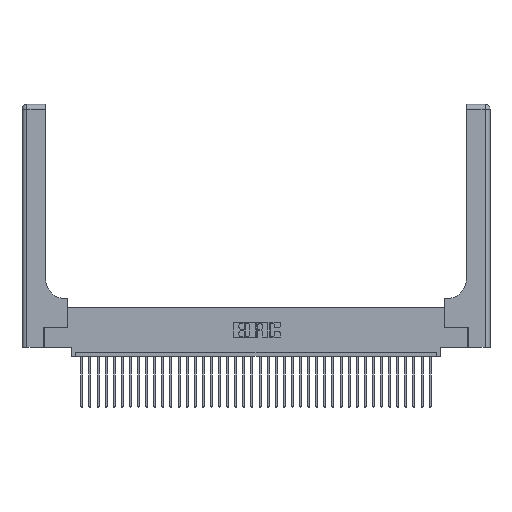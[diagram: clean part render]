
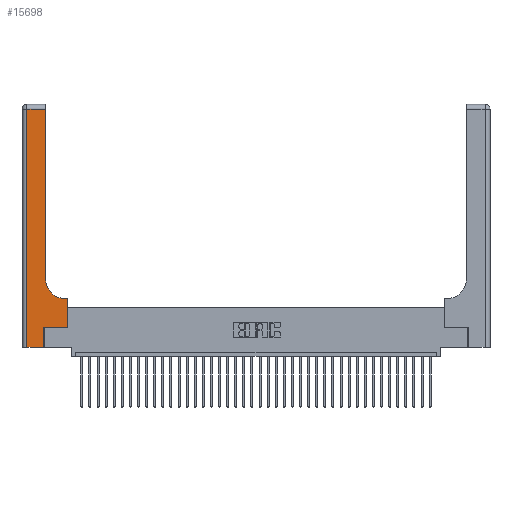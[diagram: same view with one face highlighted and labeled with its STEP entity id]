
A CAD part, top view. The second image highlights one B-rep face of the part: STEP entity #15698.
In plain terms, the highlighted planar face has unit normal (0, 0, 1).
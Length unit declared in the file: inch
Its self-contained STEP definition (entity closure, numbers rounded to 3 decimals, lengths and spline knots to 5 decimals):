
#1615 = ORIENTED_EDGE ( 'NONE', *, *, #35983, .T. ) ;
#2591 = VECTOR ( 'NONE', #10965, 39.37008 ) ;
#2613 = LINE ( 'NONE', #31323, #20630 ) ;
#2653 = CIRCLE ( 'NONE', #23347, 0.25 ) ;
#3253 = DIRECTION ( 'NONE',  ( 0., -1., 0. ) ) ;
#3875 = LINE ( 'NONE', #9169, #34372 ) ;
#4025 = CARTESIAN_POINT ( 'NONE',  ( 0.06, 2.94, 0.37 ) ) ;
#4198 = ORIENTED_EDGE ( 'NONE', *, *, #8417, .T. ) ;
#4744 = ORIENTED_EDGE ( 'NONE', *, *, #29244, .T. ) ;
#5102 = ORIENTED_EDGE ( 'NONE', *, *, #23853, .T. ) ;
#6579 = DIRECTION ( 'NONE',  ( 0., 1., 0. ) ) ;
#6632 = AXIS2_PLACEMENT_3D ( 'NONE', #10665, #25784, #16975 ) ;
#6956 = CARTESIAN_POINT ( 'NONE',  ( 0.2915, 2.94, 0.37 ) ) ;
#7447 = EDGE_CURVE ( 'NONE', #20373, #27268, #31253, .T. ) ;
#7867 = LINE ( 'NONE', #11156, #29525 ) ;
#7925 = DIRECTION ( 'NONE',  ( 0., 1., 0. ) ) ;
#7994 = CARTESIAN_POINT ( 'NONE',  ( 0., 0., 0.37 ) ) ;
#8121 = CARTESIAN_POINT ( 'NONE',  ( 0.5585, 0.25, 0.37 ) ) ;
#8356 = CARTESIAN_POINT ( 'NONE',  ( 0.269, 0.25, 0.37 ) ) ;
#8417 = EDGE_CURVE ( 'NONE', #19033, #24531, #37881, .T. ) ;
#9169 = CARTESIAN_POINT ( 'NONE',  ( 0.2915, 3., 0.37 ) ) ;
#9247 = VECTOR ( 'NONE', #31862, 39.37008 ) ;
#9699 = CARTESIAN_POINT ( 'NONE',  ( 0., 2.94, 0.37 ) ) ;
#10398 = VERTEX_POINT ( 'NONE', #6956 ) ;
#10665 = CARTESIAN_POINT ( 'NONE',  ( 0., 3., 0.37 ) ) ;
#10712 = EDGE_CURVE ( 'NONE', #16524, #20373, #2613, .T. ) ;
#10965 = DIRECTION ( 'NONE',  ( 1., 0., 0. ) ) ;
#11080 = EDGE_CURVE ( 'NONE', #20494, #18774, #17378, .T. ) ;
#11156 = CARTESIAN_POINT ( 'NONE',  ( 0.269, 0., 0.37 ) ) ;
#11181 = PLANE ( 'NONE',  #6632 ) ;
#12588 = EDGE_CURVE ( 'NONE', #24531, #20494, #32113, .T. ) ;
#12649 = DIRECTION ( 'NONE',  ( -1., 0., 0. ) ) ;
#12998 = CARTESIAN_POINT ( 'NONE',  ( 0.2915, 0.85, 0.37 ) ) ;
#14057 = VECTOR ( 'NONE', #34293, 39.37008 ) ;
#15144 = CARTESIAN_POINT ( 'NONE',  ( 0.5415, 0.6, 0.37 ) ) ;
#15698 = ADVANCED_FACE ( 'NONE', ( #36290 ), #11181, .F. ) ;
#16325 = DIRECTION ( 'NONE',  ( 0., 0., -1. ) ) ;
#16524 = VERTEX_POINT ( 'NONE', #4025 ) ;
#16700 = ORIENTED_EDGE ( 'NONE', *, *, #10712, .T. ) ;
#16975 = DIRECTION ( 'NONE',  ( -1., 0., 0. ) ) ;
#17378 = LINE ( 'NONE', #31148, #26608 ) ;
#17421 = ORIENTED_EDGE ( 'NONE', *, *, #30627, .T. ) ;
#17640 = CARTESIAN_POINT ( 'NONE',  ( 0.5585, 0.25, 0.37 ) ) ;
#18774 = VERTEX_POINT ( 'NONE', #15144 ) ;
#18900 = VERTEX_POINT ( 'NONE', #12998 ) ;
#19033 = VERTEX_POINT ( 'NONE', #27196 ) ;
#20373 = VERTEX_POINT ( 'NONE', #24460 ) ;
#20494 = VERTEX_POINT ( 'NONE', #28140 ) ;
#20630 = VECTOR ( 'NONE', #3253, 39.37008 ) ;
#22955 = LINE ( 'NONE', #9699, #30339 ) ;
#23347 = AXIS2_PLACEMENT_3D ( 'NONE', #31449, #16325, #34248 ) ;
#23853 = EDGE_CURVE ( 'NONE', #18900, #10398, #3875, .T. ) ;
#24460 = CARTESIAN_POINT ( 'NONE',  ( 0.06, 0., 0.37 ) ) ;
#24531 = VERTEX_POINT ( 'NONE', #17640 ) ;
#25506 = DIRECTION ( 'NONE',  ( -1., 0., 0. ) ) ;
#25784 = DIRECTION ( 'NONE',  ( 0., 0., -1. ) ) ;
#26002 = ORIENTED_EDGE ( 'NONE', *, *, #11080, .T. ) ;
#26049 = CARTESIAN_POINT ( 'NONE',  ( 0.269, 0., 0.37 ) ) ;
#26366 = EDGE_LOOP ( 'NONE', ( #5102, #1615, #16700, #33769, #4744, #4198, #27893, #26002, #17421 ) ) ;
#26608 = VECTOR ( 'NONE', #25506, 39.37008 ) ;
#27196 = CARTESIAN_POINT ( 'NONE',  ( 0.269, 0.25, 0.37 ) ) ;
#27268 = VERTEX_POINT ( 'NONE', #26049 ) ;
#27893 = ORIENTED_EDGE ( 'NONE', *, *, #12588, .T. ) ;
#28140 = CARTESIAN_POINT ( 'NONE',  ( 0.5585, 0.6, 0.37 ) ) ;
#29244 = EDGE_CURVE ( 'NONE', #27268, #19033, #7867, .T. ) ;
#29525 = VECTOR ( 'NONE', #7925, 39.37008 ) ;
#30339 = VECTOR ( 'NONE', #12649, 39.37008 ) ;
#30627 = EDGE_CURVE ( 'NONE', #18774, #18900, #2653, .T. ) ;
#31148 = CARTESIAN_POINT ( 'NONE',  ( 0.2915, 0.6, 0.37 ) ) ;
#31253 = LINE ( 'NONE', #7994, #2591 ) ;
#31323 = CARTESIAN_POINT ( 'NONE',  ( 0.06, 3., 0.37 ) ) ;
#31449 = CARTESIAN_POINT ( 'NONE',  ( 0.5415, 0.85, 0.37 ) ) ;
#31862 = DIRECTION ( 'NONE',  ( 1., 0., 0. ) ) ;
#32113 = LINE ( 'NONE', #8121, #14057 ) ;
#33769 = ORIENTED_EDGE ( 'NONE', *, *, #7447, .T. ) ;
#34248 = DIRECTION ( 'NONE',  ( 1., 0., 0. ) ) ;
#34293 = DIRECTION ( 'NONE',  ( 0., 1., 0. ) ) ;
#34372 = VECTOR ( 'NONE', #6579, 39.37008 ) ;
#35983 = EDGE_CURVE ( 'NONE', #10398, #16524, #22955, .T. ) ;
#36290 = FACE_OUTER_BOUND ( 'NONE', #26366, .T. ) ;
#37881 = LINE ( 'NONE', #8356, #9247 ) ;
